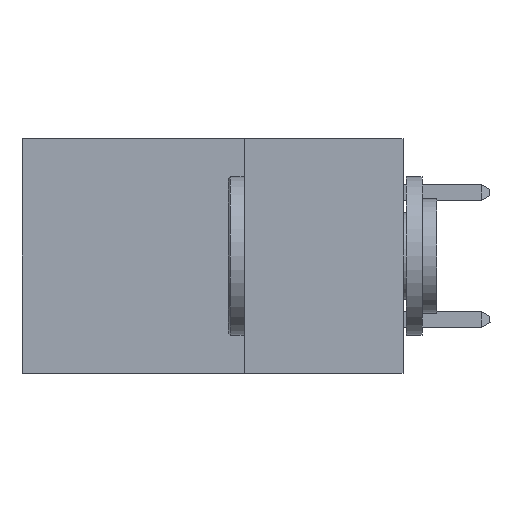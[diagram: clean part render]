
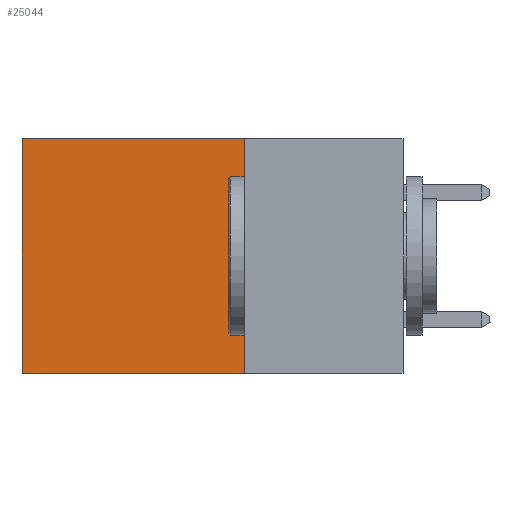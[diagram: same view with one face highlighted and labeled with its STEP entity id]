
A CAD part, left-side view. The second image highlights one B-rep face of the part: STEP entity #25044.
In plain terms, the highlighted planar face has unit normal (-1, 0, 0).
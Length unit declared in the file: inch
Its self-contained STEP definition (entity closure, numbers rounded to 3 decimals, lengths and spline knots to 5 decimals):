
#753 = DIRECTION ( 'NONE',  ( 0., 1., 0. ) ) ;
#2381 = DIRECTION ( 'NONE',  ( 0., 1., 0. ) ) ;
#2672 = VECTOR ( 'NONE', #2381, 39.37008 ) ;
#2689 = CARTESIAN_POINT ( 'NONE',  ( 0.2875, 0.25, 0. ) ) ;
#2790 = DIRECTION ( 'NONE',  ( 0., 0., -1. ) ) ;
#3414 = LINE ( 'NONE', #8619, #25003 ) ;
#3839 = VERTEX_POINT ( 'NONE', #22520 ) ;
#4580 = DIRECTION ( 'NONE',  ( 0., 0., -1. ) ) ;
#5481 = CARTESIAN_POINT ( 'NONE',  ( 0.2875, 0.6, -0.37 ) ) ;
#6115 = ORIENTED_EDGE ( 'NONE', *, *, #20177, .T. ) ;
#6557 = EDGE_LOOP ( 'NONE', ( #6115, #24163, #11592, #21050 ) ) ;
#8026 = EDGE_CURVE ( 'NONE', #3839, #14916, #24613, .T. ) ;
#8619 = CARTESIAN_POINT ( 'NONE',  ( 0.2875, 0.25, 0. ) ) ;
#11209 = DIRECTION ( 'NONE',  ( 1., 0., 0. ) ) ;
#11592 = ORIENTED_EDGE ( 'NONE', *, *, #12289, .F. ) ;
#12289 = EDGE_CURVE ( 'NONE', #25529, #3839, #3414, .T. ) ;
#14155 = VERTEX_POINT ( 'NONE', #18651 ) ;
#14916 = VERTEX_POINT ( 'NONE', #5481 ) ;
#14939 = VECTOR ( 'NONE', #753, 39.37008 ) ;
#15317 = CARTESIAN_POINT ( 'NONE',  ( 0.2875, 0.25, 0. ) ) ;
#17270 = PLANE ( 'NONE',  #22746 ) ;
#17328 = EDGE_CURVE ( 'NONE', #25529, #14155, #20519, .T. ) ;
#18651 = CARTESIAN_POINT ( 'NONE',  ( 0.2875, 0.6, 0. ) ) ;
#19304 = CARTESIAN_POINT ( 'NONE',  ( 0.2875, 0.25, -0.37 ) ) ;
#19312 = CARTESIAN_POINT ( 'NONE',  ( 0.2875, 0.6, 0. ) ) ;
#19699 = CARTESIAN_POINT ( 'NONE',  ( 0.2875, 0.25, 0. ) ) ;
#20177 = EDGE_CURVE ( 'NONE', #14155, #14916, #23251, .T. ) ;
#20519 = LINE ( 'NONE', #2689, #14939 ) ;
#20963 = DIRECTION ( 'NONE',  ( 0., 0., -1. ) ) ;
#21050 = ORIENTED_EDGE ( 'NONE', *, *, #17328, .T. ) ;
#22520 = CARTESIAN_POINT ( 'NONE',  ( 0.2875, 0.25, -0.37 ) ) ;
#22746 = AXIS2_PLACEMENT_3D ( 'NONE', #15317, #11209, #2790 ) ;
#23251 = LINE ( 'NONE', #19312, #23556 ) ;
#23556 = VECTOR ( 'NONE', #4580, 39.37008 ) ;
#24163 = ORIENTED_EDGE ( 'NONE', *, *, #8026, .F. ) ;
#24613 = LINE ( 'NONE', #19304, #2672 ) ;
#24681 = FACE_OUTER_BOUND ( 'NONE', #6557, .T. ) ;
#25003 = VECTOR ( 'NONE', #20963, 39.37008 ) ;
#25044 = ADVANCED_FACE ( 'NONE', ( #24681 ), #17270, .F. ) ;
#25529 = VERTEX_POINT ( 'NONE', #19699 ) ;
